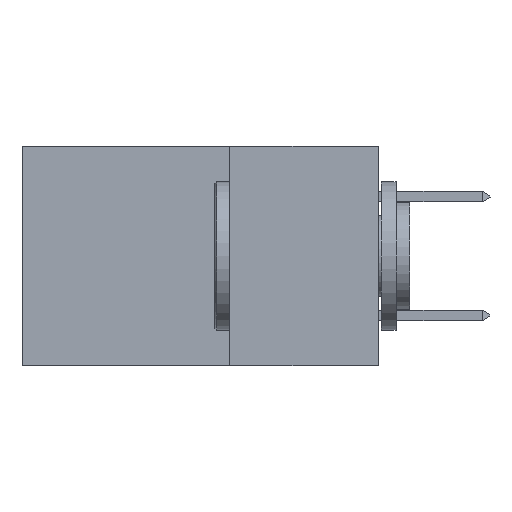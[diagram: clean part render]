
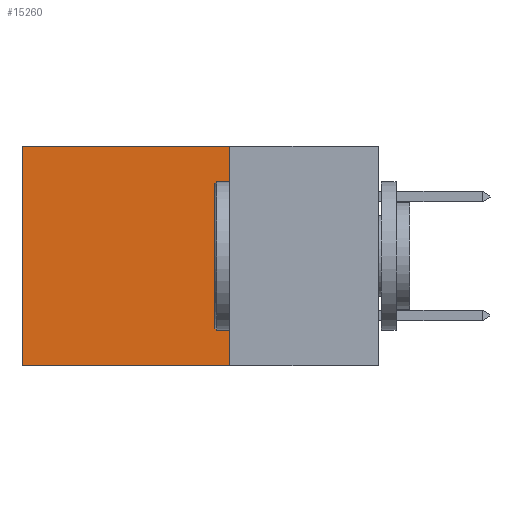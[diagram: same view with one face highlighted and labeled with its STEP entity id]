
A CAD part, left-side view. The second image highlights one B-rep face of the part: STEP entity #15260.
In plain terms, the highlighted planar face has unit normal (-1, 0, 0).
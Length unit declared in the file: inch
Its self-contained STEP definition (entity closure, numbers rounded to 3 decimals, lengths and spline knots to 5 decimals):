
#94 = PLANE ( 'NONE',  #18686 ) ;
#340 = CARTESIAN_POINT ( 'NONE',  ( 0.298, 0.6, -0.37 ) ) ;
#1005 = DIRECTION ( 'NONE',  ( 0., 1., 0. ) ) ;
#1803 = VECTOR ( 'NONE', #1005, 39.37008 ) ;
#2177 = VERTEX_POINT ( 'NONE', #18596 ) ;
#2739 = EDGE_CURVE ( 'NONE', #2177, #23344, #12858, .T. ) ;
#3382 = VERTEX_POINT ( 'NONE', #6959 ) ;
#4062 = FACE_OUTER_BOUND ( 'NONE', #17525, .T. ) ;
#5230 = LINE ( 'NONE', #14595, #16370 ) ;
#6959 = CARTESIAN_POINT ( 'NONE',  ( 0.298, 0.25, 0. ) ) ;
#9872 = CARTESIAN_POINT ( 'NONE',  ( 0.298, 0.6, 0. ) ) ;
#10379 = CARTESIAN_POINT ( 'NONE',  ( 0.298, 0.6, 0. ) ) ;
#10441 = CARTESIAN_POINT ( 'NONE',  ( 0.298, 0.25, 0. ) ) ;
#10577 = DIRECTION ( 'NONE',  ( 0., 0., -1. ) ) ;
#11265 = DIRECTION ( 'NONE',  ( 1., 0., 0. ) ) ;
#11267 = DIRECTION ( 'NONE',  ( 0., 1., 0. ) ) ;
#12018 = VECTOR ( 'NONE', #22845, 39.37008 ) ;
#12636 = VERTEX_POINT ( 'NONE', #10379 ) ;
#12858 = LINE ( 'NONE', #14717, #21942 ) ;
#13491 = LINE ( 'NONE', #9872, #12018 ) ;
#13494 = ORIENTED_EDGE ( 'NONE', *, *, #2739, .F. ) ;
#13855 = LINE ( 'NONE', #10441, #1803 ) ;
#14191 = ORIENTED_EDGE ( 'NONE', *, *, #15558, .F. ) ;
#14595 = CARTESIAN_POINT ( 'NONE',  ( 0.298, 0.25, 0. ) ) ;
#14703 = EDGE_CURVE ( 'NONE', #12636, #23344, #13491, .T. ) ;
#14717 = CARTESIAN_POINT ( 'NONE',  ( 0.298, 0.25, -0.37 ) ) ;
#15260 = ADVANCED_FACE ( 'NONE', ( #4062 ), #94, .F. ) ;
#15334 = ORIENTED_EDGE ( 'NONE', *, *, #14703, .T. ) ;
#15558 = EDGE_CURVE ( 'NONE', #3382, #2177, #5230, .T. ) ;
#16370 = VECTOR ( 'NONE', #10577, 39.37008 ) ;
#16990 = CARTESIAN_POINT ( 'NONE',  ( 0.298, 0.25, 0. ) ) ;
#17525 = EDGE_LOOP ( 'NONE', ( #15334, #13494, #14191, #21451 ) ) ;
#18596 = CARTESIAN_POINT ( 'NONE',  ( 0.298, 0.25, -0.37 ) ) ;
#18686 = AXIS2_PLACEMENT_3D ( 'NONE', #16990, #11265, #18799 ) ;
#18799 = DIRECTION ( 'NONE',  ( 0., 0., -1. ) ) ;
#19307 = EDGE_CURVE ( 'NONE', #3382, #12636, #13855, .T. ) ;
#21451 = ORIENTED_EDGE ( 'NONE', *, *, #19307, .T. ) ;
#21942 = VECTOR ( 'NONE', #11267, 39.37008 ) ;
#22845 = DIRECTION ( 'NONE',  ( 0., 0., -1. ) ) ;
#23344 = VERTEX_POINT ( 'NONE', #340 ) ;
